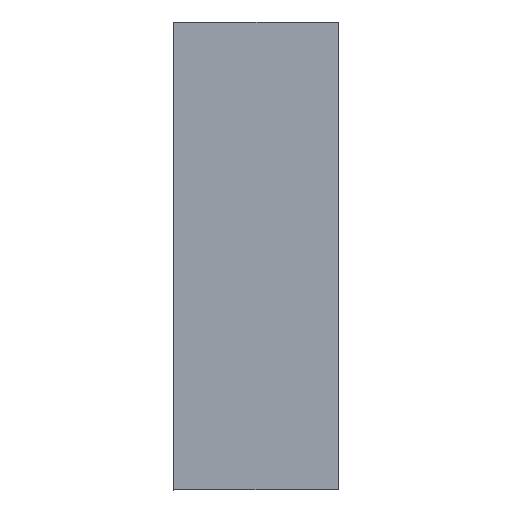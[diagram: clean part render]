
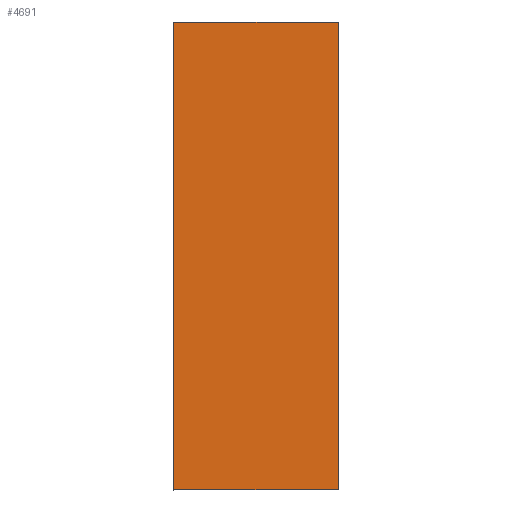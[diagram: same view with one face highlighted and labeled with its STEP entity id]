
A CAD part, front view. The second image highlights one B-rep face of the part: STEP entity #4691.
In plain terms, the highlighted planar face has unit normal (0, -1, 0).
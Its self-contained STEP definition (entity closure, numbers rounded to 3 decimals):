
#763=FACE_OUTER_BOUND('',#1075,.T.);
#1075=EDGE_LOOP('',(#3141,#3142,#3143,#3144));
#1390=LINE('',#7099,#1660);
#1393=LINE('',#7105,#1663);
#1396=LINE('',#7111,#1666);
#1399=LINE('',#7115,#1669);
#1660=VECTOR('',#5625,10.);
#1663=VECTOR('',#5630,10.);
#1666=VECTOR('',#5635,10.);
#1669=VECTOR('',#5640,10.);
#1930=VERTEX_POINT('',#7096);
#1931=VERTEX_POINT('',#7098);
#1933=VERTEX_POINT('',#7104);
#1935=VERTEX_POINT('',#7110);
#2374=EDGE_CURVE('',#1931,#1930,#1390,.T.);
#2377=EDGE_CURVE('',#1933,#1931,#1393,.T.);
#2380=EDGE_CURVE('',#1935,#1933,#1396,.T.);
#2383=EDGE_CURVE('',#1930,#1935,#1399,.T.);
#3141=ORIENTED_EDGE('',*,*,#2383,.T.);
#3142=ORIENTED_EDGE('',*,*,#2380,.T.);
#3143=ORIENTED_EDGE('',*,*,#2377,.T.);
#3144=ORIENTED_EDGE('',*,*,#2374,.T.);
#4635=PLANE('',#5023);
#4691=ADVANCED_FACE('',(#763),#4635,.T.);
#5023=AXIS2_PLACEMENT_3D('',#7116,#5641,#5642);
#5625=DIRECTION('',(0.,0.,1.));
#5630=DIRECTION('',(1.,0.,0.));
#5635=DIRECTION('',(0.,0.,-1.));
#5640=DIRECTION('',(-1.,0.,0.));
#5641=DIRECTION('center_axis',(0.,-1.,0.));
#5642=DIRECTION('ref_axis',(0.,0.,-1.));
#7096=CARTESIAN_POINT('',(12.645,-150.501,63.293));
#7098=CARTESIAN_POINT('',(12.645,-150.501,-9.309));
#7099=CARTESIAN_POINT('',(12.645,-150.501,-9.309));
#7104=CARTESIAN_POINT('',(-12.897,-150.501,-9.309));
#7105=CARTESIAN_POINT('',(-12.897,-150.501,-9.309));
#7110=CARTESIAN_POINT('',(-12.897,-150.501,63.293));
#7111=CARTESIAN_POINT('',(-12.897,-150.501,63.293));
#7115=CARTESIAN_POINT('',(12.645,-150.501,63.293));
#7116=CARTESIAN_POINT('Origin',(-0.126,-150.501,26.992));
